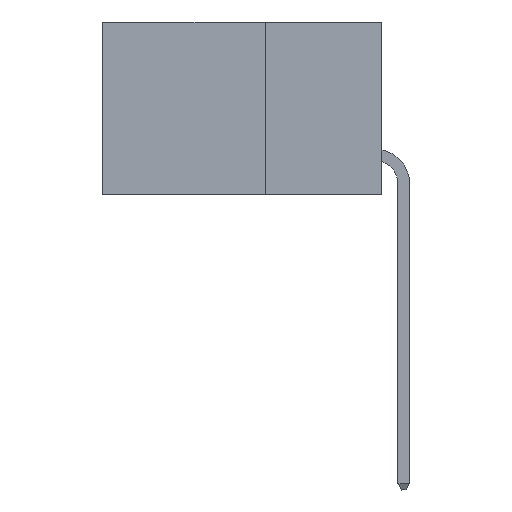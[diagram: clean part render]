
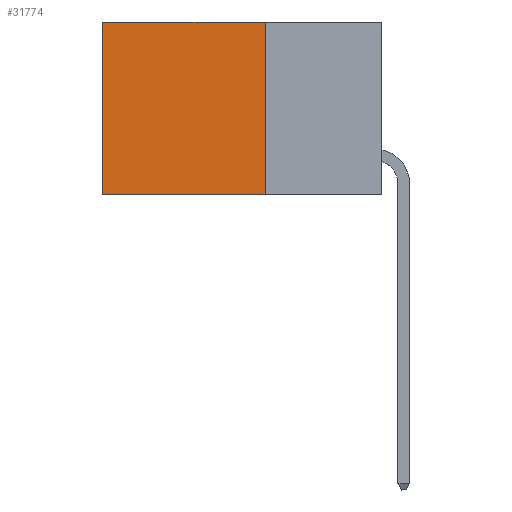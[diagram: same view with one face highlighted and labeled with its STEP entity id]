
A CAD part, left-side view. The second image highlights one B-rep face of the part: STEP entity #31774.
In plain terms, the highlighted planar face has unit normal (-1, 0, 0).
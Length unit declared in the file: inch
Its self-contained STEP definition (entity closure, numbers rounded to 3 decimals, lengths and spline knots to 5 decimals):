
#1900 = CARTESIAN_POINT ( 'NONE',  ( 0.2875, 0.6, 0. ) ) ;
#2539 = ORIENTED_EDGE ( 'NONE', *, *, #42576, .F. ) ;
#3060 = CARTESIAN_POINT ( 'NONE',  ( 0.2875, 0.25, -0.37 ) ) ;
#3581 = EDGE_CURVE ( 'NONE', #25476, #36503, #20845, .T. ) ;
#7532 = CARTESIAN_POINT ( 'NONE',  ( 0.2875, 0.25, 0. ) ) ;
#8626 = VERTEX_POINT ( 'NONE', #43997 ) ;
#11697 = LINE ( 'NONE', #36343, #12531 ) ;
#11762 = DIRECTION ( 'NONE',  ( 0., 0., -1. ) ) ;
#11988 = AXIS2_PLACEMENT_3D ( 'NONE', #39373, #15187, #11762 ) ;
#12531 = VECTOR ( 'NONE', #22186, 39.37008 ) ;
#13107 = VERTEX_POINT ( 'NONE', #41406 ) ;
#13389 = VECTOR ( 'NONE', #38416, 39.37008 ) ;
#14159 = ORIENTED_EDGE ( 'NONE', *, *, #15796, .T. ) ;
#15187 = DIRECTION ( 'NONE',  ( 1., 0., 0. ) ) ;
#15315 = EDGE_CURVE ( 'NONE', #25476, #13107, #39381, .T. ) ;
#15750 = ORIENTED_EDGE ( 'NONE', *, *, #15315, .T. ) ;
#15796 = EDGE_CURVE ( 'NONE', #13107, #8626, #22216, .T. ) ;
#20845 = LINE ( 'NONE', #21068, #13389 ) ;
#21068 = CARTESIAN_POINT ( 'NONE',  ( 0.2875, 0.25, 0. ) ) ;
#22186 = DIRECTION ( 'NONE',  ( 0., 1., 0. ) ) ;
#22216 = LINE ( 'NONE', #1900, #35491 ) ;
#22259 = FACE_OUTER_BOUND ( 'NONE', #40232, .T. ) ;
#23402 = ORIENTED_EDGE ( 'NONE', *, *, #3581, .F. ) ;
#25476 = VERTEX_POINT ( 'NONE', #7532 ) ;
#31774 = ADVANCED_FACE ( 'NONE', ( #22259 ), #32305, .F. ) ;
#32305 = PLANE ( 'NONE',  #11988 ) ;
#33215 = DIRECTION ( 'NONE',  ( 0., 1., 0. ) ) ;
#35491 = VECTOR ( 'NONE', #36145, 39.37008 ) ;
#36145 = DIRECTION ( 'NONE',  ( 0., 0., -1. ) ) ;
#36343 = CARTESIAN_POINT ( 'NONE',  ( 0.2875, 0.25, -0.37 ) ) ;
#36503 = VERTEX_POINT ( 'NONE', #3060 ) ;
#38416 = DIRECTION ( 'NONE',  ( 0., 0., -1. ) ) ;
#39373 = CARTESIAN_POINT ( 'NONE',  ( 0.2875, 0.25, 0. ) ) ;
#39381 = LINE ( 'NONE', #39838, #42784 ) ;
#39838 = CARTESIAN_POINT ( 'NONE',  ( 0.2875, 0.25, 0. ) ) ;
#40232 = EDGE_LOOP ( 'NONE', ( #14159, #2539, #23402, #15750 ) ) ;
#41406 = CARTESIAN_POINT ( 'NONE',  ( 0.2875, 0.6, 0. ) ) ;
#42576 = EDGE_CURVE ( 'NONE', #36503, #8626, #11697, .T. ) ;
#42784 = VECTOR ( 'NONE', #33215, 39.37008 ) ;
#43997 = CARTESIAN_POINT ( 'NONE',  ( 0.2875, 0.6, -0.37 ) ) ;
